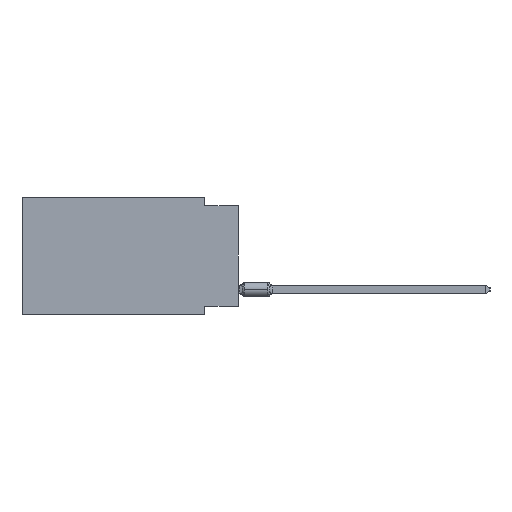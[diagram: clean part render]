
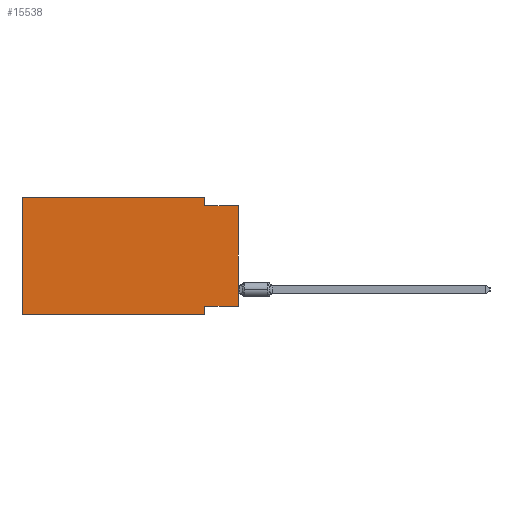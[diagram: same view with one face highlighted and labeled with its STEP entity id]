
A CAD part, left-side view. The second image highlights one B-rep face of the part: STEP entity #15538.
In plain terms, the highlighted planar face has unit normal (-1, 0, 0).
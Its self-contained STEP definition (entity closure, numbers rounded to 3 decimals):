
#591 = VECTOR ( 'NONE', #52339, 1000. ) ;
#1163 = PLANE ( 'NONE',  #58631 ) ;
#3955 = ORIENTED_EDGE ( 'NONE', *, *, #35631, .F. ) ;
#4046 = CARTESIAN_POINT ( 'NONE',  ( 0., 16.383, 0. ) ) ;
#4450 = LINE ( 'NONE', #52240, #5294 ) ;
#5153 = VERTEX_POINT ( 'NONE', #32700 ) ;
#5294 = VECTOR ( 'NONE', #24005, 1000. ) ;
#5632 = CARTESIAN_POINT ( 'NONE',  ( 0., 0., -0.635 ) ) ;
#6463 = CARTESIAN_POINT ( 'NONE',  ( 0., 16.383, 0. ) ) ;
#6524 = EDGE_CURVE ( 'NONE', #20900, #53668, #4450, .T. ) ;
#10067 = CARTESIAN_POINT ( 'NONE',  ( 0., 0., 0. ) ) ;
#10177 = VECTOR ( 'NONE', #39911, 1000. ) ;
#10548 = CARTESIAN_POINT ( 'NONE',  ( 0., 2.54, -8.89 ) ) ;
#10679 = DIRECTION ( 'NONE',  ( 0., 0., 1. ) ) ;
#11375 = LINE ( 'NONE', #25638, #10177 ) ;
#11729 = VECTOR ( 'NONE', #24805, 1000. ) ;
#13214 = EDGE_CURVE ( 'NONE', #51968, #15111, #60880, .T. ) ;
#13863 = EDGE_LOOP ( 'NONE', ( #47963, #35181, #35112, #46795, #25060, #56475, #45478, #3955 ) ) ;
#15111 = VERTEX_POINT ( 'NONE', #10548 ) ;
#15538 = ADVANCED_FACE ( 'NONE', ( #29392 ), #1163, .F. ) ;
#16436 = LINE ( 'NONE', #54621, #21490 ) ;
#17797 = CARTESIAN_POINT ( 'NONE',  ( 0., 2.54, 0. ) ) ;
#19745 = CARTESIAN_POINT ( 'NONE',  ( 0., 0., -8.255 ) ) ;
#19828 = LINE ( 'NONE', #6463, #40937 ) ;
#20900 = VERTEX_POINT ( 'NONE', #26101 ) ;
#21490 = VECTOR ( 'NONE', #30712, 1000. ) ;
#23081 = CARTESIAN_POINT ( 'NONE',  ( 0., 16.383, 0. ) ) ;
#23497 = EDGE_CURVE ( 'NONE', #53668, #58805, #19828, .T. ) ;
#23874 = LINE ( 'NONE', #24177, #11729 ) ;
#24005 = DIRECTION ( 'NONE',  ( 0., 0., 1. ) ) ;
#24177 = CARTESIAN_POINT ( 'NONE',  ( 0., 2.54, 0. ) ) ;
#24805 = DIRECTION ( 'NONE',  ( 0., 0., -1. ) ) ;
#25060 = ORIENTED_EDGE ( 'NONE', *, *, #6524, .F. ) ;
#25638 = CARTESIAN_POINT ( 'NONE',  ( 0., 16.383, -8.89 ) ) ;
#26101 = CARTESIAN_POINT ( 'NONE',  ( 0., 16.383, -8.89 ) ) ;
#26352 = VERTEX_POINT ( 'NONE', #35379 ) ;
#27955 = DIRECTION ( 'NONE',  ( 0., 0., -1. ) ) ;
#29392 = FACE_OUTER_BOUND ( 'NONE', #13863, .T. ) ;
#30712 = DIRECTION ( 'NONE',  ( 0., -1., 0. ) ) ;
#32700 = CARTESIAN_POINT ( 'NONE',  ( 0., 0., -8.255 ) ) ;
#33729 = EDGE_CURVE ( 'NONE', #58805, #26352, #23874, .T. ) ;
#33746 = CARTESIAN_POINT ( 'NONE',  ( 0., 2.54, -8.255 ) ) ;
#35112 = ORIENTED_EDGE ( 'NONE', *, *, #33729, .F. ) ;
#35181 = ORIENTED_EDGE ( 'NONE', *, *, #46642, .F. ) ;
#35379 = CARTESIAN_POINT ( 'NONE',  ( 0., 2.54, -0.635 ) ) ;
#35631 = EDGE_CURVE ( 'NONE', #5153, #51968, #51732, .T. ) ;
#36307 = DIRECTION ( 'NONE',  ( 0., 0., -1. ) ) ;
#36514 = VERTEX_POINT ( 'NONE', #5632 ) ;
#38428 = DIRECTION ( 'NONE',  ( 0., -1., 0. ) ) ;
#39911 = DIRECTION ( 'NONE',  ( 0., -1., 0. ) ) ;
#40456 = VECTOR ( 'NONE', #10679, 1000. ) ;
#40465 = CARTESIAN_POINT ( 'NONE',  ( 0., 2.54, -8.89 ) ) ;
#40569 = VECTOR ( 'NONE', #27955, 1000. ) ;
#40937 = VECTOR ( 'NONE', #38428, 1000. ) ;
#45478 = ORIENTED_EDGE ( 'NONE', *, *, #13214, .F. ) ;
#46642 = EDGE_CURVE ( 'NONE', #26352, #36514, #16436, .T. ) ;
#46795 = ORIENTED_EDGE ( 'NONE', *, *, #23497, .F. ) ;
#47963 = ORIENTED_EDGE ( 'NONE', *, *, #48182, .T. ) ;
#48182 = EDGE_CURVE ( 'NONE', #5153, #36514, #57238, .T. ) ;
#51732 = LINE ( 'NONE', #19745, #591 ) ;
#51968 = VERTEX_POINT ( 'NONE', #33746 ) ;
#52240 = CARTESIAN_POINT ( 'NONE',  ( 0., 16.383, 0. ) ) ;
#52339 = DIRECTION ( 'NONE',  ( 0., 1., 0. ) ) ;
#53668 = VERTEX_POINT ( 'NONE', #23081 ) ;
#54621 = CARTESIAN_POINT ( 'NONE',  ( 0., 0., -0.635 ) ) ;
#56475 = ORIENTED_EDGE ( 'NONE', *, *, #57084, .T. ) ;
#57084 = EDGE_CURVE ( 'NONE', #20900, #15111, #11375, .T. ) ;
#57238 = LINE ( 'NONE', #10067, #40456 ) ;
#58631 = AXIS2_PLACEMENT_3D ( 'NONE', #4046, #59652, #36307 ) ;
#58805 = VERTEX_POINT ( 'NONE', #17797 ) ;
#59652 = DIRECTION ( 'NONE',  ( 1., 0., 0. ) ) ;
#60880 = LINE ( 'NONE', #40465, #40569 ) ;
